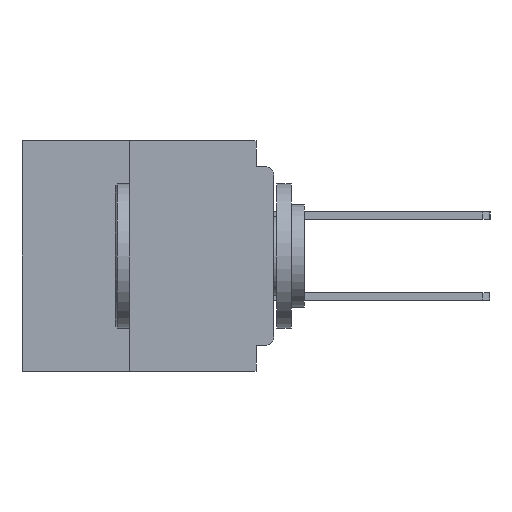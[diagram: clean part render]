
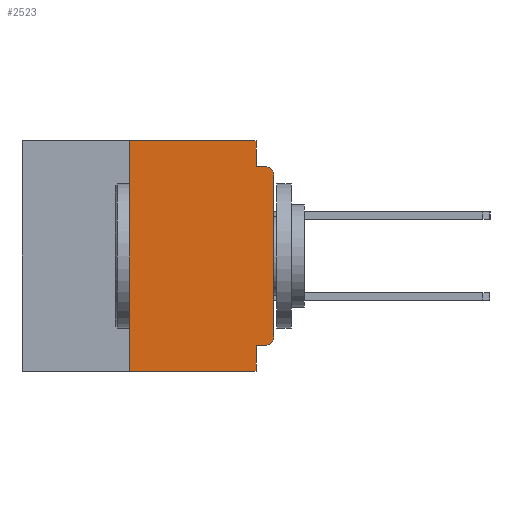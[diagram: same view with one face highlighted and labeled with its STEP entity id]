
A CAD part, left-side view. The second image highlights one B-rep face of the part: STEP entity #2523.
In plain terms, the highlighted planar face has unit normal (-1, 0, 0).
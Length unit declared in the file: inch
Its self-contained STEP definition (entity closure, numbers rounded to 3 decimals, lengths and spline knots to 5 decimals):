
#1179 = VERTEX_POINT ( 'NONE', #38838 ) ;
#1376 = DIRECTION ( 'NONE',  ( 0., -1., 0. ) ) ;
#1668 = DIRECTION ( 'NONE',  ( 0., 0., -1. ) ) ;
#1749 = ORIENTED_EDGE ( 'NONE', *, *, #12068, .T. ) ;
#2523 = ADVANCED_FACE ( 'NONE', ( #11375 ), #36410, .F. ) ;
#3056 = ORIENTED_EDGE ( 'NONE', *, *, #48979, .T. ) ;
#5470 = ORIENTED_EDGE ( 'NONE', *, *, #23864, .T. ) ;
#6253 = LINE ( 'NONE', #48653, #59626 ) ;
#6620 = CARTESIAN_POINT ( 'NONE',  ( 0., 0.437, 0. ) ) ;
#7178 = AXIS2_PLACEMENT_3D ( 'NONE', #58622, #27862, #63735 ) ;
#7758 = VERTEX_POINT ( 'NONE', #17515 ) ;
#8314 = AXIS2_PLACEMENT_3D ( 'NONE', #63589, #32930, #1668 ) ;
#8401 = VERTEX_POINT ( 'NONE', #35829 ) ;
#9254 = ORIENTED_EDGE ( 'NONE', *, *, #42701, .T. ) ;
#10399 = VERTEX_POINT ( 'NONE', #41232 ) ;
#10549 = CARTESIAN_POINT ( 'NONE',  ( 0., 0.437, -0.4 ) ) ;
#11375 = FACE_OUTER_BOUND ( 'NONE', #25921, .T. ) ;
#12068 = EDGE_CURVE ( 'NONE', #26960, #24648, #38060, .T. ) ;
#12436 = CARTESIAN_POINT ( 'NONE',  ( 0., 0.031, 0. ) ) ;
#13118 = CARTESIAN_POINT ( 'NONE',  ( 0., 0., -0.06 ) ) ;
#14752 = CARTESIAN_POINT ( 'NONE',  ( 0., 0.031, -0.045 ) ) ;
#14933 = EDGE_CURVE ( 'NONE', #51380, #1179, #47469, .T. ) ;
#15484 = LINE ( 'NONE', #44575, #38260 ) ;
#16303 = VERTEX_POINT ( 'NONE', #22892 ) ;
#16562 = ORIENTED_EDGE ( 'NONE', *, *, #14933, .F. ) ;
#17515 = CARTESIAN_POINT ( 'NONE',  ( 0., 0.031, -0.355 ) ) ;
#18208 = CARTESIAN_POINT ( 'NONE',  ( 0., 0., -0.34 ) ) ;
#19735 = EDGE_CURVE ( 'NONE', #8401, #51380, #15484, .T. ) ;
#22892 = CARTESIAN_POINT ( 'NONE',  ( 0., 0.015, -0.045 ) ) ;
#23704 = DIRECTION ( 'NONE',  ( 0., 0., 1. ) ) ;
#23864 = EDGE_CURVE ( 'NONE', #10399, #26960, #40502, .T. ) ;
#24212 = VECTOR ( 'NONE', #42958, 39.37008 ) ;
#24648 = VERTEX_POINT ( 'NONE', #13118 ) ;
#24897 = AXIS2_PLACEMENT_3D ( 'NONE', #36784, #36236, #36020 ) ;
#25921 = EDGE_LOOP ( 'NONE', ( #1749, #9254, #26009, #64902, #16562, #34577, #3056, #39924, #26436, #5470 ) ) ;
#26009 = ORIENTED_EDGE ( 'NONE', *, *, #51937, .F. ) ;
#26366 = LINE ( 'NONE', #56808, #55365 ) ;
#26436 = ORIENTED_EDGE ( 'NONE', *, *, #61512, .F. ) ;
#26960 = VERTEX_POINT ( 'NONE', #18208 ) ;
#27862 = DIRECTION ( 'NONE',  ( -1., 0., 0. ) ) ;
#31019 = DIRECTION ( 'NONE',  ( 0., -1., 0. ) ) ;
#32930 = DIRECTION ( 'NONE',  ( -1., 0., 0. ) ) ;
#34577 = ORIENTED_EDGE ( 'NONE', *, *, #19735, .F. ) ;
#35751 = LINE ( 'NONE', #10549, #61372 ) ;
#35829 = CARTESIAN_POINT ( 'NONE',  ( 0., 0.25, -0.4 ) ) ;
#36020 = DIRECTION ( 'NONE',  ( 0., 0., -1. ) ) ;
#36236 = DIRECTION ( 'NONE',  ( 1., 0., 0. ) ) ;
#36410 = PLANE ( 'NONE',  #24897 ) ;
#36784 = CARTESIAN_POINT ( 'NONE',  ( 0., 0.437, 0. ) ) ;
#38060 = LINE ( 'NONE', #63223, #24212 ) ;
#38260 = VECTOR ( 'NONE', #23704, 39.37008 ) ;
#38838 = CARTESIAN_POINT ( 'NONE',  ( 0., 0.031, 0. ) ) ;
#39833 = DIRECTION ( 'NONE',  ( 0., 0., -1. ) ) ;
#39924 = ORIENTED_EDGE ( 'NONE', *, *, #61702, .F. ) ;
#40502 = CIRCLE ( 'NONE', #7178, 0.015 ) ;
#41232 = CARTESIAN_POINT ( 'NONE',  ( 0., 0.015, -0.355 ) ) ;
#42701 = EDGE_CURVE ( 'NONE', #24648, #16303, #45286, .T. ) ;
#42875 = CARTESIAN_POINT ( 'NONE',  ( 0., 0.031, -0.4 ) ) ;
#42958 = DIRECTION ( 'NONE',  ( 0., 0., 1. ) ) ;
#43496 = VERTEX_POINT ( 'NONE', #42875 ) ;
#43808 = DIRECTION ( 'NONE',  ( 0., 0., -1. ) ) ;
#44575 = CARTESIAN_POINT ( 'NONE',  ( 0., 0.25, -0.4 ) ) ;
#45286 = CIRCLE ( 'NONE', #8314, 0.015 ) ;
#46900 = VECTOR ( 'NONE', #39833, 39.37008 ) ;
#47469 = LINE ( 'NONE', #6620, #59369 ) ;
#48489 = LINE ( 'NONE', #50381, #46900 ) ;
#48624 = CARTESIAN_POINT ( 'NONE',  ( 0., 0.25, 0. ) ) ;
#48653 = CARTESIAN_POINT ( 'NONE',  ( 0., 0., -0.355 ) ) ;
#48870 = DIRECTION ( 'NONE',  ( 0., 1., 0. ) ) ;
#48979 = EDGE_CURVE ( 'NONE', #8401, #43496, #35751, .T. ) ;
#50381 = CARTESIAN_POINT ( 'NONE',  ( 0., 0.031, -0.4 ) ) ;
#51380 = VERTEX_POINT ( 'NONE', #48624 ) ;
#51937 = EDGE_CURVE ( 'NONE', #62287, #16303, #26366, .T. ) ;
#53986 = DIRECTION ( 'NONE',  ( 0., -1., 0. ) ) ;
#55365 = VECTOR ( 'NONE', #31019, 39.37008 ) ;
#56654 = EDGE_CURVE ( 'NONE', #1179, #62287, #59064, .T. ) ;
#56808 = CARTESIAN_POINT ( 'NONE',  ( 0., 0., -0.045 ) ) ;
#57466 = VECTOR ( 'NONE', #43808, 39.37008 ) ;
#58622 = CARTESIAN_POINT ( 'NONE',  ( 0., 0.015, -0.34 ) ) ;
#59064 = LINE ( 'NONE', #12436, #57466 ) ;
#59369 = VECTOR ( 'NONE', #1376, 39.37008 ) ;
#59626 = VECTOR ( 'NONE', #48870, 39.37008 ) ;
#61372 = VECTOR ( 'NONE', #53986, 39.37008 ) ;
#61512 = EDGE_CURVE ( 'NONE', #10399, #7758, #6253, .T. ) ;
#61702 = EDGE_CURVE ( 'NONE', #7758, #43496, #48489, .T. ) ;
#62287 = VERTEX_POINT ( 'NONE', #14752 ) ;
#63223 = CARTESIAN_POINT ( 'NONE',  ( 0., 0., 0. ) ) ;
#63589 = CARTESIAN_POINT ( 'NONE',  ( 0., 0.015, -0.06 ) ) ;
#63735 = DIRECTION ( 'NONE',  ( 0., 0., -1. ) ) ;
#64902 = ORIENTED_EDGE ( 'NONE', *, *, #56654, .F. ) ;
